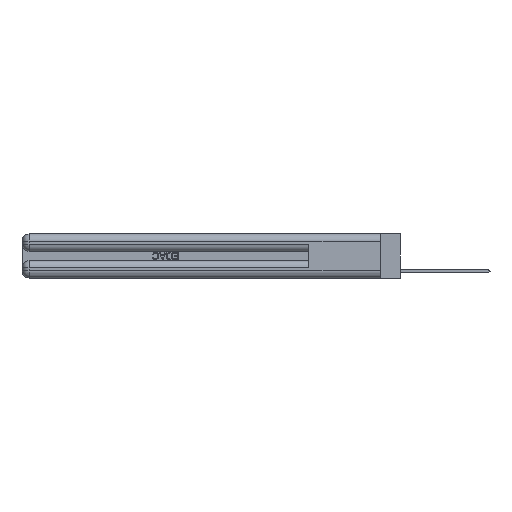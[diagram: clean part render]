
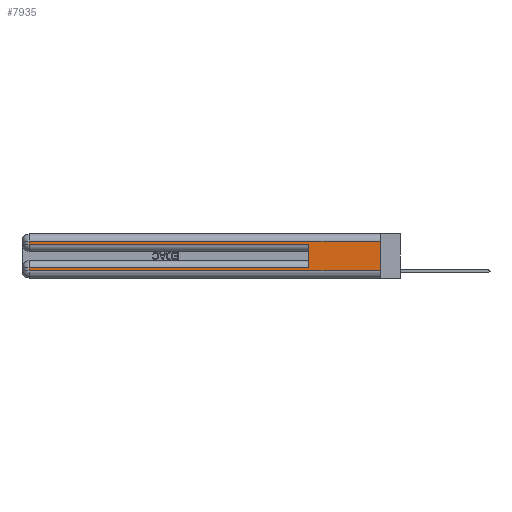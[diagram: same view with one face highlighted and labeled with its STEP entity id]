
A CAD part, left-side view. The second image highlights one B-rep face of the part: STEP entity #7935.
In plain terms, the highlighted planar face has unit normal (-1, 0, 0).
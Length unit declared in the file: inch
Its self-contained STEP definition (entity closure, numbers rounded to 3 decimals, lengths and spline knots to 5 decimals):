
#328 = DIRECTION ( 'NONE',  ( 0., 1., 0. ) ) ;
#773 = LINE ( 'NONE', #3389, #27732 ) ;
#1248 = VERTEX_POINT ( 'NONE', #31968 ) ;
#1931 = EDGE_CURVE ( 'NONE', #1248, #19098, #20934, .T. ) ;
#2542 = LINE ( 'NONE', #28264, #2844 ) ;
#2844 = VECTOR ( 'NONE', #328, 39.37008 ) ;
#3138 = LINE ( 'NONE', #32779, #20610 ) ;
#3389 = CARTESIAN_POINT ( 'NONE',  ( 0., 0., 0.285 ) ) ;
#3608 = CARTESIAN_POINT ( 'NONE',  ( 0., 0., 0.06 ) ) ;
#4043 = VERTEX_POINT ( 'NONE', #17013 ) ;
#4111 = VECTOR ( 'NONE', #15767, 39.37008 ) ;
#4126 = CARTESIAN_POINT ( 'NONE',  ( 0., 2.94, 0.06 ) ) ;
#4353 = EDGE_CURVE ( 'NONE', #19098, #24758, #21358, .T. ) ;
#4534 = LINE ( 'NONE', #10815, #4111 ) ;
#4547 = ORIENTED_EDGE ( 'NONE', *, *, #21745, .F. ) ;
#5416 = DIRECTION ( 'NONE',  ( 0., -1., 0. ) ) ;
#6693 = EDGE_CURVE ( 'NONE', #19454, #14715, #4534, .T. ) ;
#7250 = ORIENTED_EDGE ( 'NONE', *, *, #1931, .T. ) ;
#7935 = ADVANCED_FACE ( 'NONE', ( #8818 ), #10845, .F. ) ;
#8818 = FACE_OUTER_BOUND ( 'NONE', #31799, .T. ) ;
#9330 = ORIENTED_EDGE ( 'NONE', *, *, #18776, .T. ) ;
#9378 = DIRECTION ( 'NONE',  ( 0., 0., 1. ) ) ;
#10430 = ORIENTED_EDGE ( 'NONE', *, *, #6693, .F. ) ;
#10495 = CARTESIAN_POINT ( 'NONE',  ( 0., 2.94, 0.37 ) ) ;
#10815 = CARTESIAN_POINT ( 'NONE',  ( 0., 0., 0.37 ) ) ;
#10845 = PLANE ( 'NONE',  #12285 ) ;
#11959 = LINE ( 'NONE', #20953, #25817 ) ;
#12285 = AXIS2_PLACEMENT_3D ( 'NONE', #28566, #15581, #31006 ) ;
#12546 = CARTESIAN_POINT ( 'NONE',  ( 0., 0., 0.085 ) ) ;
#12683 = ORIENTED_EDGE ( 'NONE', *, *, #4353, .T. ) ;
#13030 = DIRECTION ( 'NONE',  ( 0., 0., -1. ) ) ;
#14480 = CARTESIAN_POINT ( 'NONE',  ( 0., 2.94, 0.285 ) ) ;
#14715 = VERTEX_POINT ( 'NONE', #3608 ) ;
#15072 = DIRECTION ( 'NONE',  ( 0., 1., 0. ) ) ;
#15488 = CARTESIAN_POINT ( 'NONE',  ( 0., 2.94, 0.085 ) ) ;
#15581 = DIRECTION ( 'NONE',  ( 1., 0., 0. ) ) ;
#15767 = DIRECTION ( 'NONE',  ( 0., 0., -1. ) ) ;
#16103 = ORIENTED_EDGE ( 'NONE', *, *, #23943, .T. ) ;
#16919 = VECTOR ( 'NONE', #15072, 39.37008 ) ;
#17013 = CARTESIAN_POINT ( 'NONE',  ( 0., 0.6, 0.285 ) ) ;
#17082 = VERTEX_POINT ( 'NONE', #26766 ) ;
#18535 = VECTOR ( 'NONE', #9378, 39.37008 ) ;
#18776 = EDGE_CURVE ( 'NONE', #24758, #14715, #11959, .T. ) ;
#19098 = VERTEX_POINT ( 'NONE', #15488 ) ;
#19454 = VERTEX_POINT ( 'NONE', #26671 ) ;
#20610 = VECTOR ( 'NONE', #27997, 39.37008 ) ;
#20934 = LINE ( 'NONE', #12546, #16919 ) ;
#20953 = CARTESIAN_POINT ( 'NONE',  ( 0., 0., 0.06 ) ) ;
#21358 = LINE ( 'NONE', #10495, #29289 ) ;
#21745 = EDGE_CURVE ( 'NONE', #1248, #4043, #25299, .T. ) ;
#22019 = CARTESIAN_POINT ( 'NONE',  ( 0., 0.6, 0.145 ) ) ;
#23943 = EDGE_CURVE ( 'NONE', #19454, #17082, #2542, .T. ) ;
#24575 = ORIENTED_EDGE ( 'NONE', *, *, #30067, .T. ) ;
#24758 = VERTEX_POINT ( 'NONE', #4126 ) ;
#25299 = LINE ( 'NONE', #22019, #18535 ) ;
#25817 = VECTOR ( 'NONE', #5416, 39.37008 ) ;
#26671 = CARTESIAN_POINT ( 'NONE',  ( 0., 0., 0.31 ) ) ;
#26766 = CARTESIAN_POINT ( 'NONE',  ( 0., 2.94, 0.31 ) ) ;
#27732 = VECTOR ( 'NONE', #31226, 39.37008 ) ;
#27997 = DIRECTION ( 'NONE',  ( 0., 0., -1. ) ) ;
#28264 = CARTESIAN_POINT ( 'NONE',  ( 0., 0., 0.31 ) ) ;
#28566 = CARTESIAN_POINT ( 'NONE',  ( 0., 0., 0.37 ) ) ;
#29289 = VECTOR ( 'NONE', #13030, 39.37008 ) ;
#30067 = EDGE_CURVE ( 'NONE', #32834, #4043, #773, .T. ) ;
#30297 = EDGE_CURVE ( 'NONE', #17082, #32834, #3138, .T. ) ;
#30677 = ORIENTED_EDGE ( 'NONE', *, *, #30297, .T. ) ;
#31006 = DIRECTION ( 'NONE',  ( 0., 0., -1. ) ) ;
#31226 = DIRECTION ( 'NONE',  ( 0., -1., 0. ) ) ;
#31799 = EDGE_LOOP ( 'NONE', ( #10430, #16103, #30677, #24575, #4547, #7250, #12683, #9330 ) ) ;
#31968 = CARTESIAN_POINT ( 'NONE',  ( 0., 0.6, 0.085 ) ) ;
#32779 = CARTESIAN_POINT ( 'NONE',  ( 0., 2.94, 0.37 ) ) ;
#32834 = VERTEX_POINT ( 'NONE', #14480 ) ;
